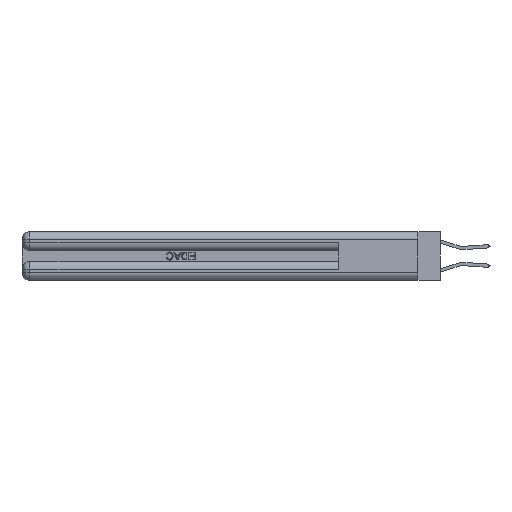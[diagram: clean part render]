
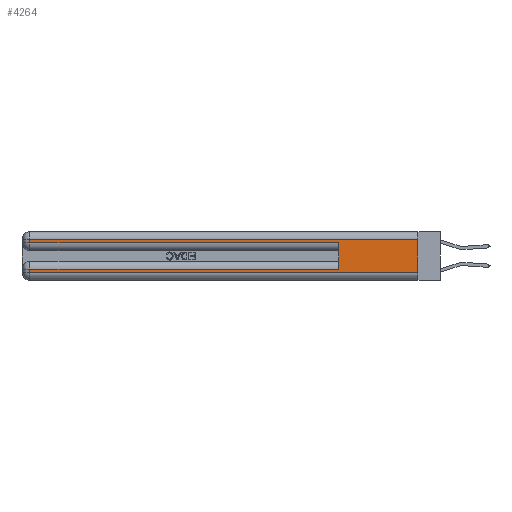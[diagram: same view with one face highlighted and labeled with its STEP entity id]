
A CAD part, left-side view. The second image highlights one B-rep face of the part: STEP entity #4264.
In plain terms, the highlighted planar face has unit normal (-1, 0, 0).
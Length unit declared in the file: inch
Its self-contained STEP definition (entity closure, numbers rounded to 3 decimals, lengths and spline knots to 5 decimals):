
#295 = EDGE_CURVE ( 'NONE', #28616, #27712, #7083, .T. ) ;
#1345 = VECTOR ( 'NONE', #12911, 39.37008 ) ;
#1725 = VECTOR ( 'NONE', #30332, 39.37008 ) ;
#1840 = AXIS2_PLACEMENT_3D ( 'NONE', #9329, #24485, #19586 ) ;
#1880 = EDGE_CURVE ( 'NONE', #28971, #29255, #24396, .T. ) ;
#2187 = CARTESIAN_POINT ( 'NONE',  ( 0., 0., 0.31 ) ) ;
#2366 = VECTOR ( 'NONE', #24406, 39.37008 ) ;
#3620 = CARTESIAN_POINT ( 'NONE',  ( 0., 0.6, 0.085 ) ) ;
#4154 = DIRECTION ( 'NONE',  ( 0., 0., -1. ) ) ;
#4264 = ADVANCED_FACE ( 'NONE', ( #32394 ), #14571, .F. ) ;
#4671 = CARTESIAN_POINT ( 'NONE',  ( 0., 0., 0.285 ) ) ;
#4804 = EDGE_CURVE ( 'NONE', #29255, #27712, #28100, .T. ) ;
#4809 = ORIENTED_EDGE ( 'NONE', *, *, #8427, .T. ) ;
#5884 = VECTOR ( 'NONE', #23093, 39.37008 ) ;
#7083 = LINE ( 'NONE', #10433, #1725 ) ;
#8427 = EDGE_CURVE ( 'NONE', #24487, #32961, #15428, .T. ) ;
#9132 = EDGE_CURVE ( 'NONE', #28616, #24487, #28468, .T. ) ;
#9329 = CARTESIAN_POINT ( 'NONE',  ( 0., 0., 0.37 ) ) ;
#10433 = CARTESIAN_POINT ( 'NONE',  ( 0., 0.6, 0.145 ) ) ;
#11086 = ORIENTED_EDGE ( 'NONE', *, *, #9132, .T. ) ;
#11491 = CARTESIAN_POINT ( 'NONE',  ( 0., 2.94, 0.31 ) ) ;
#12231 = ORIENTED_EDGE ( 'NONE', *, *, #295, .F. ) ;
#12680 = ORIENTED_EDGE ( 'NONE', *, *, #21794, .T. ) ;
#12911 = DIRECTION ( 'NONE',  ( 0., 0., -1. ) ) ;
#14166 = VERTEX_POINT ( 'NONE', #18008 ) ;
#14368 = ORIENTED_EDGE ( 'NONE', *, *, #4804, .T. ) ;
#14571 = PLANE ( 'NONE',  #1840 ) ;
#15344 = CARTESIAN_POINT ( 'NONE',  ( 0., 0., 0.085 ) ) ;
#15428 = LINE ( 'NONE', #26185, #1345 ) ;
#15931 = ORIENTED_EDGE ( 'NONE', *, *, #31235, .F. ) ;
#16096 = VECTOR ( 'NONE', #25165, 39.37008 ) ;
#17488 = CARTESIAN_POINT ( 'NONE',  ( 0., 0., 0.06 ) ) ;
#18008 = CARTESIAN_POINT ( 'NONE',  ( 0., 0., 0.31 ) ) ;
#18028 = CARTESIAN_POINT ( 'NONE',  ( 0., 2.94, 0.285 ) ) ;
#18398 = ORIENTED_EDGE ( 'NONE', *, *, #1880, .T. ) ;
#18551 = CARTESIAN_POINT ( 'NONE',  ( 0., 0.6, 0.285 ) ) ;
#19139 = VECTOR ( 'NONE', #33163, 39.37008 ) ;
#19586 = DIRECTION ( 'NONE',  ( 0., 0., -1. ) ) ;
#21794 = EDGE_CURVE ( 'NONE', #32961, #28324, #32145, .T. ) ;
#22262 = CARTESIAN_POINT ( 'NONE',  ( 0., 2.94, 0.085 ) ) ;
#22880 = DIRECTION ( 'NONE',  ( 0., -1., 0. ) ) ;
#23093 = DIRECTION ( 'NONE',  ( 0., 1., 0. ) ) ;
#23630 = VECTOR ( 'NONE', #4154, 39.37008 ) ;
#24396 = LINE ( 'NONE', #29775, #23630 ) ;
#24406 = DIRECTION ( 'NONE',  ( 0., -1., 0. ) ) ;
#24485 = DIRECTION ( 'NONE',  ( 1., 0., 0. ) ) ;
#24487 = VERTEX_POINT ( 'NONE', #22262 ) ;
#25165 = DIRECTION ( 'NONE',  ( 0., 0., -1. ) ) ;
#25348 = CARTESIAN_POINT ( 'NONE',  ( 0., 0., 0.37 ) ) ;
#26185 = CARTESIAN_POINT ( 'NONE',  ( 0., 2.94, 0.37 ) ) ;
#26308 = VECTOR ( 'NONE', #22880, 39.37008 ) ;
#26941 = CARTESIAN_POINT ( 'NONE',  ( 0., 0., 0.06 ) ) ;
#27637 = LINE ( 'NONE', #2187, #5884 ) ;
#27712 = VERTEX_POINT ( 'NONE', #18551 ) ;
#28100 = LINE ( 'NONE', #4671, #26308 ) ;
#28324 = VERTEX_POINT ( 'NONE', #17488 ) ;
#28418 = ORIENTED_EDGE ( 'NONE', *, *, #29956, .T. ) ;
#28468 = LINE ( 'NONE', #15344, #19139 ) ;
#28616 = VERTEX_POINT ( 'NONE', #3620 ) ;
#28971 = VERTEX_POINT ( 'NONE', #11491 ) ;
#29255 = VERTEX_POINT ( 'NONE', #18028 ) ;
#29537 = EDGE_LOOP ( 'NONE', ( #15931, #28418, #18398, #14368, #12231, #11086, #4809, #12680 ) ) ;
#29775 = CARTESIAN_POINT ( 'NONE',  ( 0., 2.94, 0.37 ) ) ;
#29956 = EDGE_CURVE ( 'NONE', #14166, #28971, #27637, .T. ) ;
#30332 = DIRECTION ( 'NONE',  ( 0., 0., 1. ) ) ;
#31235 = EDGE_CURVE ( 'NONE', #14166, #28324, #33055, .T. ) ;
#31389 = CARTESIAN_POINT ( 'NONE',  ( 0., 2.94, 0.06 ) ) ;
#32145 = LINE ( 'NONE', #26941, #2366 ) ;
#32394 = FACE_OUTER_BOUND ( 'NONE', #29537, .T. ) ;
#32961 = VERTEX_POINT ( 'NONE', #31389 ) ;
#33055 = LINE ( 'NONE', #25348, #16096 ) ;
#33163 = DIRECTION ( 'NONE',  ( 0., 1., 0. ) ) ;
